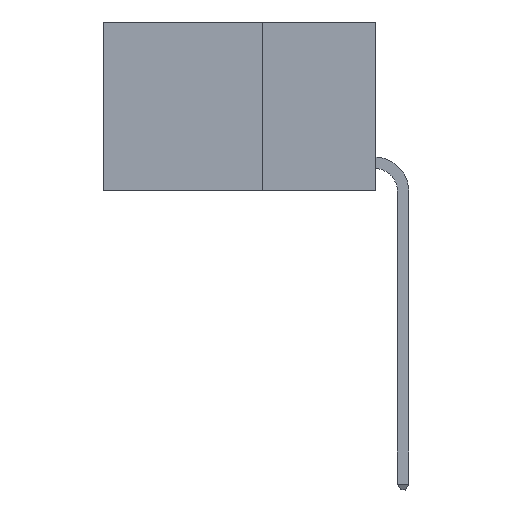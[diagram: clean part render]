
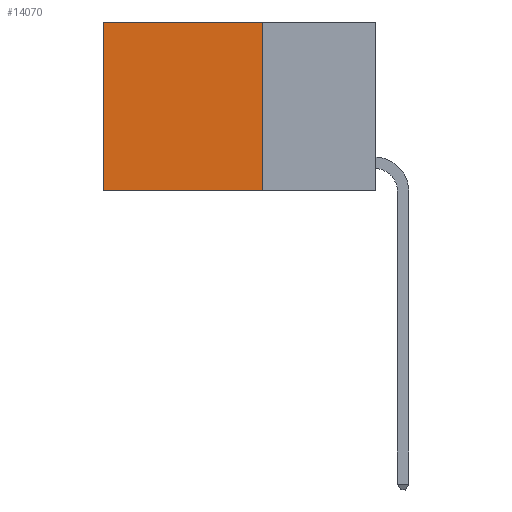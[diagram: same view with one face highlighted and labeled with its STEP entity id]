
A CAD part, left-side view. The second image highlights one B-rep face of the part: STEP entity #14070.
In plain terms, the highlighted planar face has unit normal (-1, 0, 0).
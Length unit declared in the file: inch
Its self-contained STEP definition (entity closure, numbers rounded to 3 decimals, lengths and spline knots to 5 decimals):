
#213 = VERTEX_POINT ( 'NONE', #19731 ) ;
#247 = VECTOR ( 'NONE', #20972, 39.37008 ) ;
#500 = LINE ( 'NONE', #11666, #17316 ) ;
#655 = EDGE_CURVE ( 'NONE', #213, #5518, #1520, .T. ) ;
#854 = ORIENTED_EDGE ( 'NONE', *, *, #655, .F. ) ;
#1078 = PLANE ( 'NONE',  #3807 ) ;
#1520 = LINE ( 'NONE', #21462, #4117 ) ;
#1894 = VERTEX_POINT ( 'NONE', #3533 ) ;
#2923 = CARTESIAN_POINT ( 'NONE',  ( 0.2625, 0.25, -0.37 ) ) ;
#3325 = CARTESIAN_POINT ( 'NONE',  ( 0.2625, 0.25, 0. ) ) ;
#3482 = ORIENTED_EDGE ( 'NONE', *, *, #12476, .T. ) ;
#3533 = CARTESIAN_POINT ( 'NONE',  ( 0.2625, 0.6, 0. ) ) ;
#3807 = AXIS2_PLACEMENT_3D ( 'NONE', #9512, #18066, #21228 ) ;
#4117 = VECTOR ( 'NONE', #18091, 39.37008 ) ;
#5518 = VERTEX_POINT ( 'NONE', #2923 ) ;
#6385 = CARTESIAN_POINT ( 'NONE',  ( 0.2625, 0.6, 0. ) ) ;
#6694 = LINE ( 'NONE', #3325, #9911 ) ;
#8830 = EDGE_LOOP ( 'NONE', ( #18278, #10347, #854, #3482 ) ) ;
#9512 = CARTESIAN_POINT ( 'NONE',  ( 0.2625, 0.25, 0. ) ) ;
#9911 = VECTOR ( 'NONE', #13392, 39.37008 ) ;
#10116 = EDGE_CURVE ( 'NONE', #1894, #15091, #18002, .T. ) ;
#10347 = ORIENTED_EDGE ( 'NONE', *, *, #10408, .F. ) ;
#10408 = EDGE_CURVE ( 'NONE', #5518, #15091, #500, .T. ) ;
#11666 = CARTESIAN_POINT ( 'NONE',  ( 0.2625, 0.25, -0.37 ) ) ;
#12476 = EDGE_CURVE ( 'NONE', #213, #1894, #6694, .T. ) ;
#13392 = DIRECTION ( 'NONE',  ( 0., 1., 0. ) ) ;
#13768 = CARTESIAN_POINT ( 'NONE',  ( 0.2625, 0.6, -0.37 ) ) ;
#14070 = ADVANCED_FACE ( 'NONE', ( #15991 ), #1078, .F. ) ;
#15091 = VERTEX_POINT ( 'NONE', #13768 ) ;
#15991 = FACE_OUTER_BOUND ( 'NONE', #8830, .T. ) ;
#16913 = DIRECTION ( 'NONE',  ( 0., 1., 0. ) ) ;
#17316 = VECTOR ( 'NONE', #16913, 39.37008 ) ;
#18002 = LINE ( 'NONE', #6385, #247 ) ;
#18066 = DIRECTION ( 'NONE',  ( 1., 0., 0. ) ) ;
#18091 = DIRECTION ( 'NONE',  ( 0., 0., -1. ) ) ;
#18278 = ORIENTED_EDGE ( 'NONE', *, *, #10116, .T. ) ;
#19731 = CARTESIAN_POINT ( 'NONE',  ( 0.2625, 0.25, 0. ) ) ;
#20972 = DIRECTION ( 'NONE',  ( 0., 0., -1. ) ) ;
#21228 = DIRECTION ( 'NONE',  ( 0., 0., -1. ) ) ;
#21462 = CARTESIAN_POINT ( 'NONE',  ( 0.2625, 0.25, 0. ) ) ;
